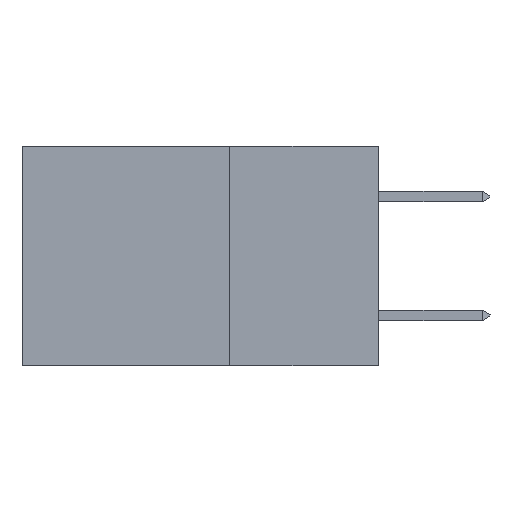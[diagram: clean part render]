
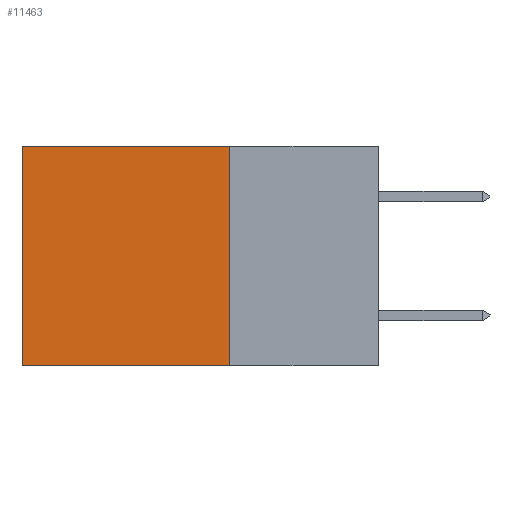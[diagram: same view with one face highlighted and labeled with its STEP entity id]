
A CAD part, left-side view. The second image highlights one B-rep face of the part: STEP entity #11463.
In plain terms, the highlighted planar face has unit normal (-1, 0, 0).
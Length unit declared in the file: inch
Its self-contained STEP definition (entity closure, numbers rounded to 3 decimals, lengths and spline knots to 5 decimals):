
#570 = DIRECTION ( 'NONE',  ( 0., 1., 0. ) ) ;
#1366 = VECTOR ( 'NONE', #6864, 39.37008 ) ;
#1954 = LINE ( 'NONE', #11682, #12671 ) ;
#2099 = ORIENTED_EDGE ( 'NONE', *, *, #12894, .F. ) ;
#2457 = CARTESIAN_POINT ( 'NONE',  ( 0.298, 0.6, 0. ) ) ;
#2727 = VERTEX_POINT ( 'NONE', #6481 ) ;
#3127 = ORIENTED_EDGE ( 'NONE', *, *, #7716, .T. ) ;
#3677 = DIRECTION ( 'NONE',  ( 0., 0., -1. ) ) ;
#4323 = VECTOR ( 'NONE', #570, 39.37008 ) ;
#4554 = VERTEX_POINT ( 'NONE', #4949 ) ;
#4633 = PLANE ( 'NONE',  #5734 ) ;
#4949 = CARTESIAN_POINT ( 'NONE',  ( 0.298, 0.6, -0.37 ) ) ;
#5408 = LINE ( 'NONE', #2457, #14053 ) ;
#5734 = AXIS2_PLACEMENT_3D ( 'NONE', #15194, #7272, #9965 ) ;
#6481 = CARTESIAN_POINT ( 'NONE',  ( 0.298, 0.25, -0.37 ) ) ;
#6864 = DIRECTION ( 'NONE',  ( 0., 1., 0. ) ) ;
#7272 = DIRECTION ( 'NONE',  ( 1., 0., 0. ) ) ;
#7716 = EDGE_CURVE ( 'NONE', #9705, #11786, #14846, .T. ) ;
#8948 = CARTESIAN_POINT ( 'NONE',  ( 0.298, 0.25, 0. ) ) ;
#9705 = VERTEX_POINT ( 'NONE', #8948 ) ;
#9965 = DIRECTION ( 'NONE',  ( 0., 0., -1. ) ) ;
#10646 = EDGE_CURVE ( 'NONE', #9705, #2727, #1954, .T. ) ;
#10741 = CARTESIAN_POINT ( 'NONE',  ( 0.298, 0.25, -0.37 ) ) ;
#11306 = EDGE_LOOP ( 'NONE', ( #13290, #2099, #11838, #3127 ) ) ;
#11463 = ADVANCED_FACE ( 'NONE', ( #12842 ), #4633, .F. ) ;
#11682 = CARTESIAN_POINT ( 'NONE',  ( 0.298, 0.25, 0. ) ) ;
#11739 = DIRECTION ( 'NONE',  ( 0., 0., -1. ) ) ;
#11786 = VERTEX_POINT ( 'NONE', #14081 ) ;
#11838 = ORIENTED_EDGE ( 'NONE', *, *, #10646, .F. ) ;
#12671 = VECTOR ( 'NONE', #11739, 39.37008 ) ;
#12842 = FACE_OUTER_BOUND ( 'NONE', #11306, .T. ) ;
#12894 = EDGE_CURVE ( 'NONE', #2727, #4554, #14778, .T. ) ;
#13290 = ORIENTED_EDGE ( 'NONE', *, *, #15706, .T. ) ;
#14053 = VECTOR ( 'NONE', #3677, 39.37008 ) ;
#14081 = CARTESIAN_POINT ( 'NONE',  ( 0.298, 0.6, 0. ) ) ;
#14778 = LINE ( 'NONE', #10741, #1366 ) ;
#14846 = LINE ( 'NONE', #16333, #4323 ) ;
#15194 = CARTESIAN_POINT ( 'NONE',  ( 0.298, 0.25, 0. ) ) ;
#15706 = EDGE_CURVE ( 'NONE', #11786, #4554, #5408, .T. ) ;
#16333 = CARTESIAN_POINT ( 'NONE',  ( 0.298, 0.25, 0. ) ) ;
